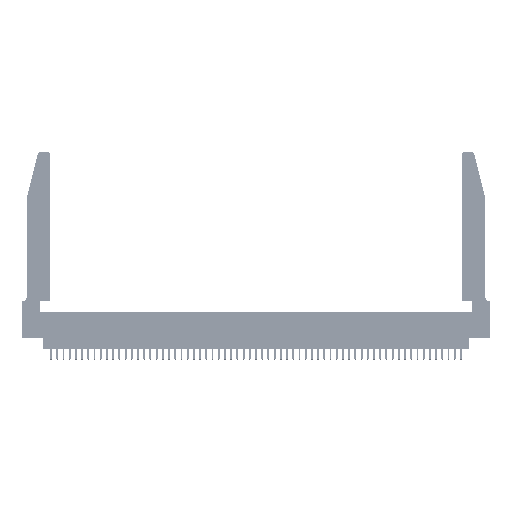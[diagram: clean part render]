
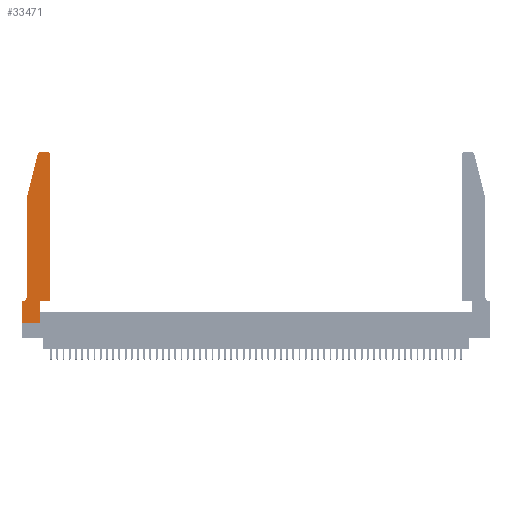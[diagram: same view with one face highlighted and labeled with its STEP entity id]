
A CAD part, top view. The second image highlights one B-rep face of the part: STEP entity #33471.
In plain terms, the highlighted planar face has unit normal (0, 0, 1).
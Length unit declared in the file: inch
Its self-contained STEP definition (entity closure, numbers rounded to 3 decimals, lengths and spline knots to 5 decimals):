
#155 = CARTESIAN_POINT ( 'NONE',  ( 0.0755, 0.42, 0.37 ) ) ;
#1543 = EDGE_CURVE ( 'NONE', #35997, #48875, #13507, .T. ) ;
#2051 = VECTOR ( 'NONE', #7976, 39.37008 ) ;
#3737 = ORIENTED_EDGE ( 'NONE', *, *, #15081, .T. ) ;
#3981 = EDGE_CURVE ( 'NONE', #39399, #5904, #50694, .T. ) ;
#4004 = EDGE_CURVE ( 'NONE', #21968, #52392, #40880, .T. ) ;
#5032 = DIRECTION ( 'NONE',  ( 1., 0., 0. ) ) ;
#5142 = CARTESIAN_POINT ( 'NONE',  ( 0.0755, 0.35, 0.37 ) ) ;
#5904 = VERTEX_POINT ( 'NONE', #37620 ) ;
#7512 = EDGE_CURVE ( 'NONE', #5904, #35997, #18838, .T. ) ;
#7976 = DIRECTION ( 'NONE',  ( 0., -1., 0. ) ) ;
#8938 = VECTOR ( 'NONE', #38188, 39.37008 ) ;
#8965 = DIRECTION ( 'NONE',  ( -1., 0., 0. ) ) ;
#8980 = DIRECTION ( 'NONE',  ( 0., -1., 0. ) ) ;
#9605 = CARTESIAN_POINT ( 'NONE',  ( 0.4505, 0.35, 0.37 ) ) ;
#9918 = LINE ( 'NONE', #41105, #2051 ) ;
#10781 = AXIS2_PLACEMENT_3D ( 'NONE', #46405, #17267, #25671 ) ;
#11393 = VECTOR ( 'NONE', #43684, 39.37008 ) ;
#11856 = LINE ( 'NONE', #13025, #31504 ) ;
#11920 = ORIENTED_EDGE ( 'NONE', *, *, #7512, .T. ) ;
#11974 = DIRECTION ( 'NONE',  ( 0., 1., 0. ) ) ;
#12593 = DIRECTION ( 'NONE',  ( -1., 0., 0. ) ) ;
#13025 = CARTESIAN_POINT ( 'NONE',  ( 0., 0., 0.37 ) ) ;
#13507 = LINE ( 'NONE', #42387, #8938 ) ;
#13726 = DIRECTION ( 'NONE',  ( 1., 0., 0. ) ) ;
#15022 = ORIENTED_EDGE ( 'NONE', *, *, #15971, .T. ) ;
#15081 = EDGE_CURVE ( 'NONE', #49500, #45047, #19997, .T. ) ;
#15194 = ORIENTED_EDGE ( 'NONE', *, *, #49774, .T. ) ;
#15684 = CARTESIAN_POINT ( 'NONE',  ( 0., 0.35, 0.37 ) ) ;
#15971 = EDGE_CURVE ( 'NONE', #45047, #17155, #53352, .T. ) ;
#16154 = CARTESIAN_POINT ( 'NONE',  ( 0.2865, 0.35, 0.37 ) ) ;
#17155 = VERTEX_POINT ( 'NONE', #29797 ) ;
#17267 = DIRECTION ( 'NONE',  ( 0., 0., 1. ) ) ;
#17531 = EDGE_CURVE ( 'NONE', #17155, #30057, #9918, .T. ) ;
#18627 = CARTESIAN_POINT ( 'NONE',  ( 0.284, 2.75, 0.37 ) ) ;
#18838 = LINE ( 'NONE', #16154, #23389 ) ;
#19997 = CIRCLE ( 'NONE', #51149, 0.03 ) ;
#20121 = FACE_OUTER_BOUND ( 'NONE', #42376, .T. ) ;
#21826 = DIRECTION ( 'NONE',  ( 1., 0., 0. ) ) ;
#21968 = VERTEX_POINT ( 'NONE', #26653 ) ;
#23389 = VECTOR ( 'NONE', #11974, 39.37008 ) ;
#23713 = CARTESIAN_POINT ( 'NONE',  ( 0.2865, 0.35, 0.37 ) ) ;
#25440 = LINE ( 'NONE', #50674, #48383 ) ;
#25671 = DIRECTION ( 'NONE',  ( 1., 0., 0. ) ) ;
#26073 = EDGE_CURVE ( 'NONE', #49632, #39399, #11856, .T. ) ;
#26232 = DIRECTION ( 'NONE',  ( 0., 0., 1. ) ) ;
#26653 = CARTESIAN_POINT ( 'NONE',  ( 0.4505, 2.72, 0.37 ) ) ;
#27100 = ORIENTED_EDGE ( 'NONE', *, *, #52506, .T. ) ;
#27214 = CARTESIAN_POINT ( 'NONE',  ( 0.25487, 2.72718, 0.37 ) ) ;
#27492 = CARTESIAN_POINT ( 'NONE',  ( 0.4505, 0.35, 0.37 ) ) ;
#27636 = ORIENTED_EDGE ( 'NONE', *, *, #17531, .T. ) ;
#29378 = ORIENTED_EDGE ( 'NONE', *, *, #26073, .T. ) ;
#29797 = CARTESIAN_POINT ( 'NONE',  ( 0.0755, 2., 0.37 ) ) ;
#30054 = DIRECTION ( 'NONE',  ( 0., 0., 1. ) ) ;
#30057 = VERTEX_POINT ( 'NONE', #155 ) ;
#30394 = CARTESIAN_POINT ( 'NONE',  ( 0.284, 2.72, 0.37 ) ) ;
#30692 = DIRECTION ( 'NONE',  ( 0., 1., 0. ) ) ;
#31061 = VECTOR ( 'NONE', #5032, 39.37008 ) ;
#31166 = CARTESIAN_POINT ( 'NONE',  ( 0., 0., 0.37 ) ) ;
#31316 = EDGE_CURVE ( 'NONE', #46836, #49632, #41487, .T. ) ;
#31504 = VECTOR ( 'NONE', #8980, 39.37008 ) ;
#33464 = DIRECTION ( 'NONE',  ( 0., 0., -1. ) ) ;
#33471 = ADVANCED_FACE ( 'NONE', ( #20121 ), #42191, .T. ) ;
#33794 = CARTESIAN_POINT ( 'NONE',  ( 0., 0., 0.37 ) ) ;
#34939 = VECTOR ( 'NONE', #8965, 39.37008 ) ;
#35026 = AXIS2_PLACEMENT_3D ( 'NONE', #42906, #26232, #21826 ) ;
#35997 = VERTEX_POINT ( 'NONE', #23713 ) ;
#36995 = ORIENTED_EDGE ( 'NONE', *, *, #31316, .T. ) ;
#37306 = CARTESIAN_POINT ( 'NONE',  ( 0.4205, 2.75, 0.37 ) ) ;
#37620 = CARTESIAN_POINT ( 'NONE',  ( 0.2865, 0., 0.37 ) ) ;
#37846 = VECTOR ( 'NONE', #30692, 39.37008 ) ;
#38188 = DIRECTION ( 'NONE',  ( 1., 0., 0. ) ) ;
#39399 = VERTEX_POINT ( 'NONE', #31166 ) ;
#39692 = CARTESIAN_POINT ( 'NONE',  ( 0.0055, 0.35, 0.37 ) ) ;
#39996 = CIRCLE ( 'NONE', #40213, 0.07 ) ;
#40021 = CARTESIAN_POINT ( 'NONE',  ( 0.0755, 2., 0.37 ) ) ;
#40213 = AXIS2_PLACEMENT_3D ( 'NONE', #46247, #33464, #42207 ) ;
#40880 = CIRCLE ( 'NONE', #35026, 0.03 ) ;
#41105 = CARTESIAN_POINT ( 'NONE',  ( 0.0755, 2., 0.37 ) ) ;
#41487 = LINE ( 'NONE', #5142, #34939 ) ;
#42191 = PLANE ( 'NONE',  #10781 ) ;
#42207 = DIRECTION ( 'NONE',  ( -1., 0., 0. ) ) ;
#42376 = EDGE_LOOP ( 'NONE', ( #15194, #3737, #15022, #27636, #27100, #36995, #29378, #52751, #11920, #50942, #50756, #43882 ) ) ;
#42387 = CARTESIAN_POINT ( 'NONE',  ( 0.4505, 0.35, 0.37 ) ) ;
#42906 = CARTESIAN_POINT ( 'NONE',  ( 0.4205, 2.72, 0.37 ) ) ;
#43684 = DIRECTION ( 'NONE',  ( -0.239, -0.971, 0. ) ) ;
#43882 = ORIENTED_EDGE ( 'NONE', *, *, #4004, .T. ) ;
#45047 = VERTEX_POINT ( 'NONE', #27214 ) ;
#46247 = CARTESIAN_POINT ( 'NONE',  ( 0.0055, 0.42, 0.37 ) ) ;
#46405 = CARTESIAN_POINT ( 'NONE',  ( 0., 0.35, 0.37 ) ) ;
#46836 = VERTEX_POINT ( 'NONE', #39692 ) ;
#48383 = VECTOR ( 'NONE', #12593, 39.37008 ) ;
#48875 = VERTEX_POINT ( 'NONE', #27492 ) ;
#49500 = VERTEX_POINT ( 'NONE', #18627 ) ;
#49632 = VERTEX_POINT ( 'NONE', #15684 ) ;
#49774 = EDGE_CURVE ( 'NONE', #52392, #49500, #25440, .T. ) ;
#50674 = CARTESIAN_POINT ( 'NONE',  ( 0.2605, 2.75, 0.37 ) ) ;
#50694 = LINE ( 'NONE', #33794, #31061 ) ;
#50756 = ORIENTED_EDGE ( 'NONE', *, *, #50768, .T. ) ;
#50768 = EDGE_CURVE ( 'NONE', #48875, #21968, #51601, .T. ) ;
#50942 = ORIENTED_EDGE ( 'NONE', *, *, #1543, .T. ) ;
#51149 = AXIS2_PLACEMENT_3D ( 'NONE', #30394, #30054, #13726 ) ;
#51601 = LINE ( 'NONE', #9605, #37846 ) ;
#52392 = VERTEX_POINT ( 'NONE', #37306 ) ;
#52506 = EDGE_CURVE ( 'NONE', #30057, #46836, #39996, .T. ) ;
#52751 = ORIENTED_EDGE ( 'NONE', *, *, #3981, .T. ) ;
#53352 = LINE ( 'NONE', #40021, #11393 ) ;
